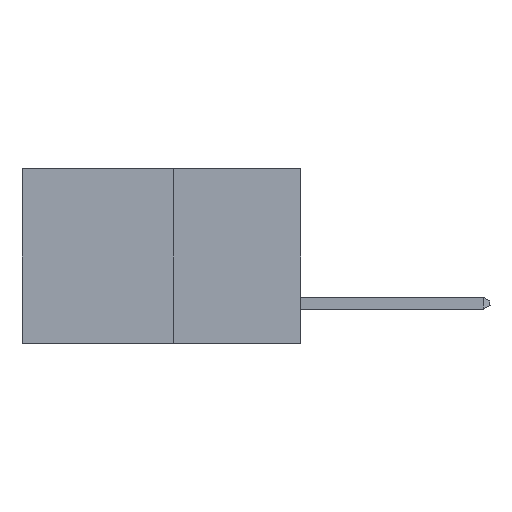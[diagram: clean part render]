
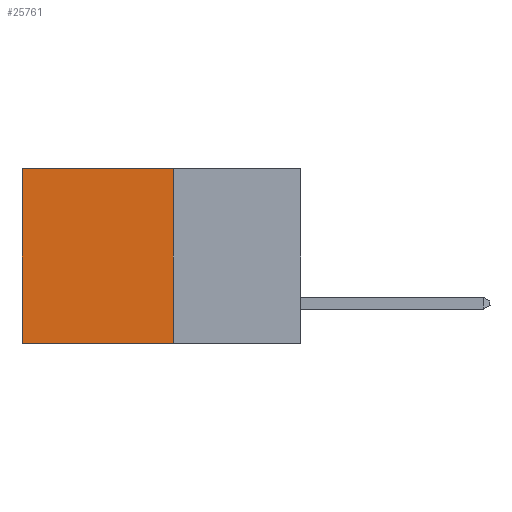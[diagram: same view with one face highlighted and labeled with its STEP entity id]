
A CAD part, left-side view. The second image highlights one B-rep face of the part: STEP entity #25761.
In plain terms, the highlighted planar face has unit normal (-1, 0, 0).
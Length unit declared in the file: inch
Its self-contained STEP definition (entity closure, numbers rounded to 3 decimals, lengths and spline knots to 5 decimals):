
#468 = VERTEX_POINT ( 'NONE', #5368 ) ;
#1423 = ORIENTED_EDGE ( 'NONE', *, *, #9891, .T. ) ;
#2063 = EDGE_CURVE ( 'NONE', #15578, #16812, #15141, .T. ) ;
#3800 = VECTOR ( 'NONE', #20110, 39.37008 ) ;
#4071 = ORIENTED_EDGE ( 'NONE', *, *, #15828, .F. ) ;
#4158 = EDGE_LOOP ( 'NONE', ( #23495, #21156, #4071, #1423 ) ) ;
#4272 = CARTESIAN_POINT ( 'NONE',  ( 0.277, 0.27, -0.37 ) ) ;
#4800 = LINE ( 'NONE', #16643, #14792 ) ;
#5368 = CARTESIAN_POINT ( 'NONE',  ( 0.277, 0.59, 0. ) ) ;
#5394 = VECTOR ( 'NONE', #9096, 39.37008 ) ;
#8059 = EDGE_CURVE ( 'NONE', #468, #16812, #4800, .T. ) ;
#9096 = DIRECTION ( 'NONE',  ( 0., 1., 0. ) ) ;
#9546 = CARTESIAN_POINT ( 'NONE',  ( 0.277, 0.59, -0.37 ) ) ;
#9891 = EDGE_CURVE ( 'NONE', #21648, #468, #16711, .T. ) ;
#10338 = DIRECTION ( 'NONE',  ( 0., 0., -1. ) ) ;
#10606 = CARTESIAN_POINT ( 'NONE',  ( 0.277, 0.27, -0.37 ) ) ;
#10733 = DIRECTION ( 'NONE',  ( 1., 0., 0. ) ) ;
#11299 = LINE ( 'NONE', #10606, #21949 ) ;
#11530 = FACE_OUTER_BOUND ( 'NONE', #4158, .T. ) ;
#12867 = CARTESIAN_POINT ( 'NONE',  ( 0.277, 0.27, 0. ) ) ;
#14792 = VECTOR ( 'NONE', #10338, 39.37008 ) ;
#15141 = LINE ( 'NONE', #25010, #3800 ) ;
#15578 = VERTEX_POINT ( 'NONE', #24705 ) ;
#15828 = EDGE_CURVE ( 'NONE', #21648, #15578, #11299, .T. ) ;
#16643 = CARTESIAN_POINT ( 'NONE',  ( 0.277, 0.59, -0.37 ) ) ;
#16711 = LINE ( 'NONE', #23919, #5394 ) ;
#16812 = VERTEX_POINT ( 'NONE', #9546 ) ;
#19151 = DIRECTION ( 'NONE',  ( 0., 0., -1. ) ) ;
#20110 = DIRECTION ( 'NONE',  ( 0., 1., 0. ) ) ;
#21156 = ORIENTED_EDGE ( 'NONE', *, *, #2063, .F. ) ;
#21229 = PLANE ( 'NONE',  #25395 ) ;
#21648 = VERTEX_POINT ( 'NONE', #12867 ) ;
#21949 = VECTOR ( 'NONE', #19151, 39.37008 ) ;
#23495 = ORIENTED_EDGE ( 'NONE', *, *, #8059, .T. ) ;
#23919 = CARTESIAN_POINT ( 'NONE',  ( 0.277, 0.27, 0. ) ) ;
#24705 = CARTESIAN_POINT ( 'NONE',  ( 0.277, 0.27, -0.37 ) ) ;
#25010 = CARTESIAN_POINT ( 'NONE',  ( 0.277, 0.27, -0.37 ) ) ;
#25395 = AXIS2_PLACEMENT_3D ( 'NONE', #4272, #10733, #25546 ) ;
#25546 = DIRECTION ( 'NONE',  ( 0., 0., -1. ) ) ;
#25761 = ADVANCED_FACE ( 'NONE', ( #11530 ), #21229, .F. ) ;
